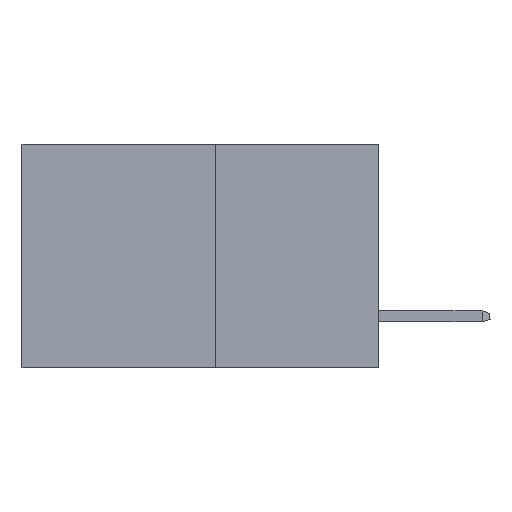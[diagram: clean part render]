
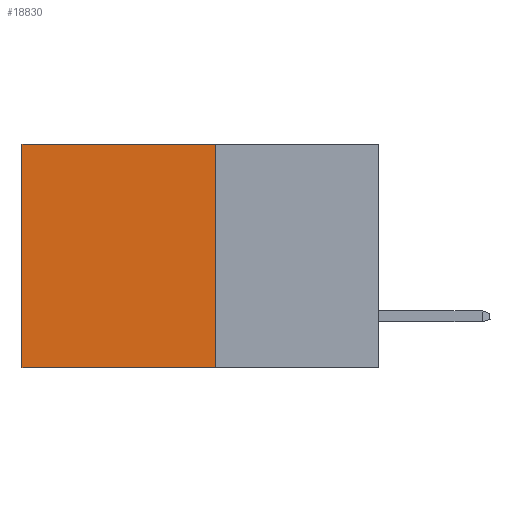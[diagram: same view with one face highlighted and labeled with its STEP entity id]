
A CAD part, left-side view. The second image highlights one B-rep face of the part: STEP entity #18830.
In plain terms, the highlighted planar face has unit normal (-1, 0, 0).
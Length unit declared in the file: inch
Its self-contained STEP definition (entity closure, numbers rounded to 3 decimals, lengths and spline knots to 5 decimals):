
#320 = VECTOR ( 'NONE', #2099, 39.37008 ) ;
#845 = EDGE_CURVE ( 'NONE', #18864, #8737, #13557, .T. ) ;
#2099 = DIRECTION ( 'NONE',  ( 0., 1., 0. ) ) ;
#2242 = CARTESIAN_POINT ( 'NONE',  ( 0.277, 0.27, 0. ) ) ;
#2546 = EDGE_CURVE ( 'NONE', #18864, #7244, #2973, .T. ) ;
#2973 = LINE ( 'NONE', #7018, #15237 ) ;
#3700 = ORIENTED_EDGE ( 'NONE', *, *, #9033, .T. ) ;
#4177 = DIRECTION ( 'NONE',  ( 0., 0., -1. ) ) ;
#4252 = EDGE_CURVE ( 'NONE', #7244, #9438, #17469, .T. ) ;
#7018 = CARTESIAN_POINT ( 'NONE',  ( 0.277, 0.27, -0.37 ) ) ;
#7244 = VERTEX_POINT ( 'NONE', #12759 ) ;
#7461 = CARTESIAN_POINT ( 'NONE',  ( 0.277, 0.27, -0.37 ) ) ;
#8105 = CARTESIAN_POINT ( 'NONE',  ( 0.277, 0.59, -0.37 ) ) ;
#8132 = EDGE_LOOP ( 'NONE', ( #3700, #18991, #20330, #16695 ) ) ;
#8668 = VECTOR ( 'NONE', #11984, 39.37008 ) ;
#8737 = VERTEX_POINT ( 'NONE', #16511 ) ;
#9033 = EDGE_CURVE ( 'NONE', #8737, #9438, #12554, .T. ) ;
#9438 = VERTEX_POINT ( 'NONE', #8105 ) ;
#11984 = DIRECTION ( 'NONE',  ( 0., 1., 0. ) ) ;
#12516 = PLANE ( 'NONE',  #16674 ) ;
#12554 = LINE ( 'NONE', #14841, #20686 ) ;
#12759 = CARTESIAN_POINT ( 'NONE',  ( 0.277, 0.27, -0.37 ) ) ;
#13036 = CARTESIAN_POINT ( 'NONE',  ( 0.277, 0.27, -0.37 ) ) ;
#13557 = LINE ( 'NONE', #2242, #320 ) ;
#13894 = DIRECTION ( 'NONE',  ( 0., 0., -1. ) ) ;
#14175 = DIRECTION ( 'NONE',  ( 1., 0., 0. ) ) ;
#14244 = CARTESIAN_POINT ( 'NONE',  ( 0.277, 0.27, 0. ) ) ;
#14417 = FACE_OUTER_BOUND ( 'NONE', #8132, .T. ) ;
#14764 = DIRECTION ( 'NONE',  ( 0., 0., -1. ) ) ;
#14841 = CARTESIAN_POINT ( 'NONE',  ( 0.277, 0.59, -0.37 ) ) ;
#15237 = VECTOR ( 'NONE', #13894, 39.37008 ) ;
#16511 = CARTESIAN_POINT ( 'NONE',  ( 0.277, 0.59, 0. ) ) ;
#16674 = AXIS2_PLACEMENT_3D ( 'NONE', #7461, #14175, #4177 ) ;
#16695 = ORIENTED_EDGE ( 'NONE', *, *, #845, .T. ) ;
#17469 = LINE ( 'NONE', #13036, #8668 ) ;
#18830 = ADVANCED_FACE ( 'NONE', ( #14417 ), #12516, .F. ) ;
#18864 = VERTEX_POINT ( 'NONE', #14244 ) ;
#18991 = ORIENTED_EDGE ( 'NONE', *, *, #4252, .F. ) ;
#20330 = ORIENTED_EDGE ( 'NONE', *, *, #2546, .F. ) ;
#20686 = VECTOR ( 'NONE', #14764, 39.37008 ) ;
